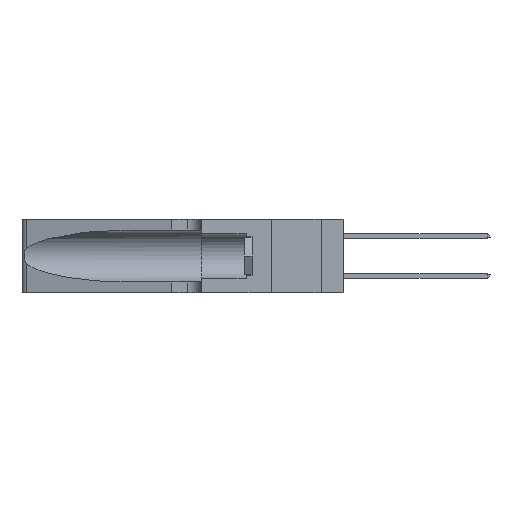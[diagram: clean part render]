
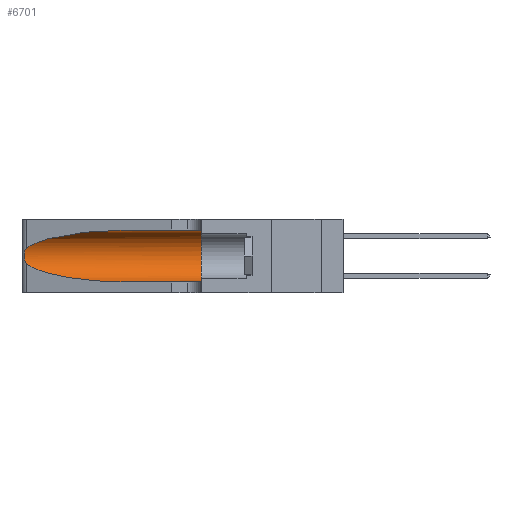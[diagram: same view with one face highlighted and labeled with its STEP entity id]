
A CAD part, left-side view. The second image highlights one B-rep face of the part: STEP entity #6701.
In plain terms, the highlighted cylindrical face has radius 3.308 mm (diameter 6.617 mm), a partial arc.
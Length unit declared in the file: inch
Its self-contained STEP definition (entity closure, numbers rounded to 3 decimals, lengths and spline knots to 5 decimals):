
#309 = DIRECTION ( 'NONE',  ( 0., -1., 0. ) ) ;
#345 = EDGE_CURVE ( 'NONE', #6096, #3865, #21489, .T. ) ;
#665 = CARTESIAN_POINT ( 'NONE',  ( 0.26017, 1.23833, 0.17102 ) ) ;
#893 = CYLINDRICAL_SURFACE ( 'NONE', #3393, 0.13025 ) ;
#1114 = VECTOR ( 'NONE', #19387, 39.37008 ) ;
#1525 = FACE_OUTER_BOUND ( 'NONE', #9803, .T. ) ;
#1588 = CARTESIAN_POINT ( 'NONE',  ( 0.18966, 0.96281, 0.31525 ) ) ;
#1683 = CARTESIAN_POINT ( 'NONE',  ( 0.25487, 1.22718, 0.22369 ) ) ;
#2687 = CARTESIAN_POINT ( 'NONE',  ( 0.25789, 1.23486, 0.15765 ) ) ;
#3030 = VERTEX_POINT ( 'NONE', #16212 ) ;
#3273 = B_SPLINE_CURVE_WITH_KNOTS ( 'NONE', 3,
 ( #6612, #16518, #18484, #8618, #22332, #10639, #24283, #12628, #665, #14618, #2687, #16605, #4666, #18572 ),
 .UNSPECIFIED., .F., .F.,
 ( 4, 2, 2, 2, 2, 2, 4 ),
 ( 0., 0.00027, 0.00053, 0.00107, 0.0016, 0.00187, 0.00214 ),
 .UNSPECIFIED. ) ;
#3393 = AXIS2_PLACEMENT_3D ( 'NONE', #21924, #309, #16187 ) ;
#3865 = VERTEX_POINT ( 'NONE', #16961 ) ;
#4666 = CARTESIAN_POINT ( 'NONE',  ( 0.25555, 1.22993, 0.14849 ) ) ;
#6096 = VERTEX_POINT ( 'NONE', #15403 ) ;
#6612 = CARTESIAN_POINT ( 'NONE',  ( 0.25487, 1.22718, 0.22369 ) ) ;
#6701 = ADVANCED_FACE ( 'NONE', ( #1525 ), #893, .F. ) ;
#7521 = ORIENTED_EDGE ( 'NONE', *, *, #8884, .T. ) ;
#8476 = ORIENTED_EDGE ( 'NONE', *, *, #345, .F. ) ;
#8540 = EDGE_CURVE ( 'NONE', #3865, #3030, #16410, .T. ) ;
#8618 = CARTESIAN_POINT ( 'NONE',  ( 0.25787, 1.23484, 0.2124 ) ) ;
#8884 = EDGE_CURVE ( 'NONE', #12143, #22342, #3273, .T. ) ;
#9102 = CARTESIAN_POINT ( 'NONE',  ( 0.1305, 0.72297, 0.05475 ) ) ;
#9738 = CARTESIAN_POINT ( 'NONE',  ( 0.2373, 1.15595, 0.08982 ) ) ;
#9803 = EDGE_LOOP ( 'NONE', ( #17529, #7521, #16713, #10582, #24814, #8476 ) ) ;
#10582 = ORIENTED_EDGE ( 'NONE', *, *, #20565, .T. ) ;
#10639 = CARTESIAN_POINT ( 'NONE',  ( 0.26018, 1.23835, 0.19895 ) ) ;
#11608 = DIRECTION ( 'NONE',  ( 0., 1., 0. ) ) ;
#11629 = AXIS2_PLACEMENT_3D ( 'NONE', #23284, #11608, #25218 ) ;
#11630 = CARTESIAN_POINT ( 'NONE',  ( 0.1305, 0.72297, 0.31525 ) ) ;
#12143 = VERTEX_POINT ( 'NONE', #18460 ) ;
#12628 = CARTESIAN_POINT ( 'NONE',  ( 0.26075, 1.23896, 0.178 ) ) ;
#13334 =( BOUNDED_CURVE ( )  B_SPLINE_CURVE ( 3, ( #11630, #1588, #13599, #1683 ),
 .UNSPECIFIED., .F., .F. ) 
 B_SPLINE_CURVE_WITH_KNOTS ( ( 4, 4 ),
 ( 1.5708, 2.84003 ),
 .UNSPECIFIED. ) 
 CURVE ( )  GEOMETRIC_REPRESENTATION_ITEM ( )  RATIONAL_B_SPLINE_CURVE ( ( 1., 0.87, 0.87, 1. ) ) 
 REPRESENTATION_ITEM ( '' )  );
#13599 = CARTESIAN_POINT ( 'NONE',  ( 0.2373, 1.15595, 0.28018 ) ) ;
#13716 = CARTESIAN_POINT ( 'NONE',  ( 0.1305, 0.72297, 0.05475 ) ) ;
#14618 = CARTESIAN_POINT ( 'NONE',  ( 0.25856, 1.23593, 0.16098 ) ) ;
#15403 = CARTESIAN_POINT ( 'NONE',  ( 0.1305, 0.72297, 0.31525 ) ) ;
#16187 = DIRECTION ( 'NONE',  ( 0., 0., -1. ) ) ;
#16212 = CARTESIAN_POINT ( 'NONE',  ( 0.1305, 0.35, 0.05475 ) ) ;
#16349 = VECTOR ( 'NONE', #23821, 39.37008 ) ;
#16410 = CIRCLE ( 'NONE', #11629, 0.13025 ) ;
#16518 = CARTESIAN_POINT ( 'NONE',  ( 0.25555, 1.22994, 0.2215 ) ) ;
#16605 = CARTESIAN_POINT ( 'NONE',  ( 0.25639, 1.23186, 0.15144 ) ) ;
#16713 = ORIENTED_EDGE ( 'NONE', *, *, #24649, .T. ) ;
#16961 = CARTESIAN_POINT ( 'NONE',  ( 0.1305, 0.35, 0.31525 ) ) ;
#16990 = LINE ( 'NONE', #17445, #1114 ) ;
#17445 = CARTESIAN_POINT ( 'NONE',  ( 0.1305, 1.61858, 0.05475 ) ) ;
#17529 = ORIENTED_EDGE ( 'NONE', *, *, #25236, .T. ) ;
#18460 = CARTESIAN_POINT ( 'NONE',  ( 0.25487, 1.22718, 0.22369 ) ) ;
#18484 = CARTESIAN_POINT ( 'NONE',  ( 0.25639, 1.23184, 0.21858 ) ) ;
#18572 = CARTESIAN_POINT ( 'NONE',  ( 0.25487, 1.22718, 0.14631 ) ) ;
#19387 = DIRECTION ( 'NONE',  ( 0., -1., 0. ) ) ;
#19547 = CARTESIAN_POINT ( 'NONE',  ( 0.25487, 1.22718, 0.14631 ) ) ;
#20106 = CARTESIAN_POINT ( 'NONE',  ( 0.1305, 1.61858, 0.31525 ) ) ;
#20565 = EDGE_CURVE ( 'NONE', #23332, #3030, #16990, .T. ) ;
#21489 = LINE ( 'NONE', #20106, #16349 ) ;
#21573 = CARTESIAN_POINT ( 'NONE',  ( 0.25487, 1.22718, 0.14631 ) ) ;
#21924 = CARTESIAN_POINT ( 'NONE',  ( 0.1305, 1.61858, 0.185 ) ) ;
#22332 = CARTESIAN_POINT ( 'NONE',  ( 0.25854, 1.2359, 0.20912 ) ) ;
#22342 = VERTEX_POINT ( 'NONE', #21573 ) ;
#22381 =( BOUNDED_CURVE ( )  B_SPLINE_CURVE ( 3, ( #19547, #9738, #25355, #13716 ),
 .UNSPECIFIED., .F., .T. ) 
 B_SPLINE_CURVE_WITH_KNOTS ( ( 4, 4 ),
 ( 3.44316, 4.71239 ),
 .UNSPECIFIED. ) 
 CURVE ( )  GEOMETRIC_REPRESENTATION_ITEM ( )  RATIONAL_B_SPLINE_CURVE ( ( 1., 0.87, 0.87, 1. ) ) 
 REPRESENTATION_ITEM ( '' )  );
#23284 = CARTESIAN_POINT ( 'NONE',  ( 0.1305, 0.35, 0.185 ) ) ;
#23332 = VERTEX_POINT ( 'NONE', #9102 ) ;
#23821 = DIRECTION ( 'NONE',  ( 0., -1., 0. ) ) ;
#24283 = CARTESIAN_POINT ( 'NONE',  ( 0.26075, 1.23896, 0.19203 ) ) ;
#24649 = EDGE_CURVE ( 'NONE', #22342, #23332, #22381, .T. ) ;
#24814 = ORIENTED_EDGE ( 'NONE', *, *, #8540, .F. ) ;
#25218 = DIRECTION ( 'NONE',  ( 0., 0., 1. ) ) ;
#25236 = EDGE_CURVE ( 'NONE', #6096, #12143, #13334, .T. ) ;
#25355 = CARTESIAN_POINT ( 'NONE',  ( 0.18966, 0.96281, 0.05475 ) ) ;
